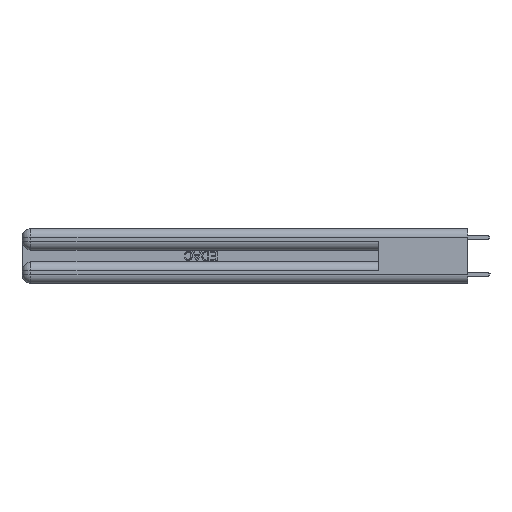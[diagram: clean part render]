
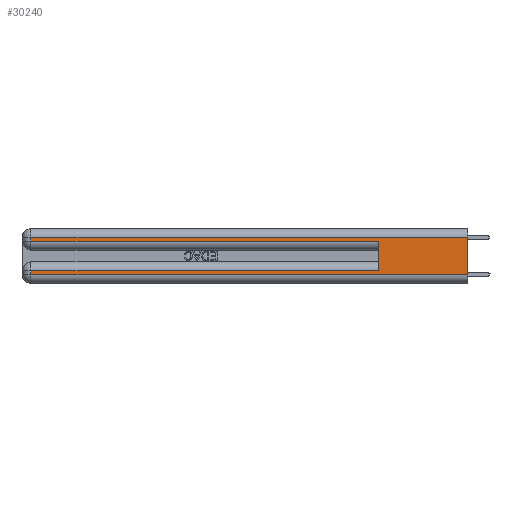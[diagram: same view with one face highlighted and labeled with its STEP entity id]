
A CAD part, left-side view. The second image highlights one B-rep face of the part: STEP entity #30240.
In plain terms, the highlighted planar face has unit normal (-1, 0, 0).
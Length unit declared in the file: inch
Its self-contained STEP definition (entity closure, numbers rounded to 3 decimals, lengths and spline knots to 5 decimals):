
#7 = CARTESIAN_POINT ( 'NONE',  ( 0., 2.94, 0.37 ) ) ;
#3219 = CARTESIAN_POINT ( 'NONE',  ( 0., 0., 0.085 ) ) ;
#3755 = EDGE_CURVE ( 'NONE', #18527, #27031, #7612, .T. ) ;
#4106 = AXIS2_PLACEMENT_3D ( 'NONE', #27947, #5730, #11053 ) ;
#4420 = CARTESIAN_POINT ( 'NONE',  ( 0., 2.94, 0.285 ) ) ;
#5433 = EDGE_CURVE ( 'NONE', #17912, #18527, #13097, .T. ) ;
#5436 = VECTOR ( 'NONE', #29998, 39.37008 ) ;
#5730 = DIRECTION ( 'NONE',  ( 1., 0., 0. ) ) ;
#5735 = CARTESIAN_POINT ( 'NONE',  ( 0., 2.94, 0.31 ) ) ;
#6537 = VECTOR ( 'NONE', #25739, 39.37008 ) ;
#6724 = DIRECTION ( 'NONE',  ( 0., -1., 0. ) ) ;
#6914 = EDGE_LOOP ( 'NONE', ( #13247, #14036, #29151, #11154, #9798, #8799, #14814, #30757 ) ) ;
#7612 = LINE ( 'NONE', #7, #22036 ) ;
#7779 = VECTOR ( 'NONE', #24035, 39.37008 ) ;
#7890 = VECTOR ( 'NONE', #28165, 39.37008 ) ;
#7951 = CARTESIAN_POINT ( 'NONE',  ( 0., 0., 0.31 ) ) ;
#8275 = LINE ( 'NONE', #7951, #5436 ) ;
#8799 = ORIENTED_EDGE ( 'NONE', *, *, #5433, .T. ) ;
#9798 = ORIENTED_EDGE ( 'NONE', *, *, #31322, .F. ) ;
#9923 = VERTEX_POINT ( 'NONE', #28962 ) ;
#10013 = CARTESIAN_POINT ( 'NONE',  ( 0., 2.94, 0.37 ) ) ;
#10562 = VERTEX_POINT ( 'NONE', #21533 ) ;
#11053 = DIRECTION ( 'NONE',  ( 0., 0., -1. ) ) ;
#11154 = ORIENTED_EDGE ( 'NONE', *, *, #29884, .T. ) ;
#12151 = EDGE_CURVE ( 'NONE', #27031, #10562, #17333, .T. ) ;
#12779 = DIRECTION ( 'NONE',  ( 0., 0., -1. ) ) ;
#13097 = LINE ( 'NONE', #3219, #6537 ) ;
#13236 = LINE ( 'NONE', #25394, #7890 ) ;
#13247 = ORIENTED_EDGE ( 'NONE', *, *, #23794, .F. ) ;
#13486 = FACE_OUTER_BOUND ( 'NONE', #6914, .T. ) ;
#13489 = VERTEX_POINT ( 'NONE', #31961 ) ;
#14008 = CARTESIAN_POINT ( 'NONE',  ( 0., 0., 0.285 ) ) ;
#14036 = ORIENTED_EDGE ( 'NONE', *, *, #27481, .T. ) ;
#14279 = CARTESIAN_POINT ( 'NONE',  ( 0., 0., 0.06 ) ) ;
#14561 = VERTEX_POINT ( 'NONE', #5735 ) ;
#14814 = ORIENTED_EDGE ( 'NONE', *, *, #3755, .T. ) ;
#15209 = EDGE_CURVE ( 'NONE', #14561, #22999, #19588, .T. ) ;
#16082 = CARTESIAN_POINT ( 'NONE',  ( 0., 2.94, 0.085 ) ) ;
#17333 = LINE ( 'NONE', #14279, #31464 ) ;
#17912 = VERTEX_POINT ( 'NONE', #22678 ) ;
#18527 = VERTEX_POINT ( 'NONE', #16082 ) ;
#19588 = LINE ( 'NONE', #10013, #20721 ) ;
#19607 = DIRECTION ( 'NONE',  ( 0., 0., -1. ) ) ;
#20479 = PLANE ( 'NONE',  #4106 ) ;
#20721 = VECTOR ( 'NONE', #12779, 39.37008 ) ;
#21533 = CARTESIAN_POINT ( 'NONE',  ( 0., 0., 0.06 ) ) ;
#22036 = VECTOR ( 'NONE', #19607, 39.37008 ) ;
#22073 = CARTESIAN_POINT ( 'NONE',  ( 0., 0.6, 0.145 ) ) ;
#22678 = CARTESIAN_POINT ( 'NONE',  ( 0., 0.6, 0.085 ) ) ;
#22899 = CARTESIAN_POINT ( 'NONE',  ( 0., 2.94, 0.06 ) ) ;
#22999 = VERTEX_POINT ( 'NONE', #4420 ) ;
#23243 = VECTOR ( 'NONE', #6724, 39.37008 ) ;
#23794 = EDGE_CURVE ( 'NONE', #13489, #10562, #13236, .T. ) ;
#24035 = DIRECTION ( 'NONE',  ( 0., 0., 1. ) ) ;
#24648 = DIRECTION ( 'NONE',  ( 0., -1., 0. ) ) ;
#25394 = CARTESIAN_POINT ( 'NONE',  ( 0., 0., 0.37 ) ) ;
#25739 = DIRECTION ( 'NONE',  ( 0., 1., 0. ) ) ;
#27031 = VERTEX_POINT ( 'NONE', #22899 ) ;
#27481 = EDGE_CURVE ( 'NONE', #13489, #14561, #8275, .T. ) ;
#27947 = CARTESIAN_POINT ( 'NONE',  ( 0., 0., 0.37 ) ) ;
#28165 = DIRECTION ( 'NONE',  ( 0., 0., -1. ) ) ;
#28962 = CARTESIAN_POINT ( 'NONE',  ( 0., 0.6, 0.285 ) ) ;
#29151 = ORIENTED_EDGE ( 'NONE', *, *, #15209, .T. ) ;
#29217 = LINE ( 'NONE', #22073, #7779 ) ;
#29884 = EDGE_CURVE ( 'NONE', #22999, #9923, #31376, .T. ) ;
#29998 = DIRECTION ( 'NONE',  ( 0., 1., 0. ) ) ;
#30240 = ADVANCED_FACE ( 'NONE', ( #13486 ), #20479, .F. ) ;
#30757 = ORIENTED_EDGE ( 'NONE', *, *, #12151, .T. ) ;
#31322 = EDGE_CURVE ( 'NONE', #17912, #9923, #29217, .T. ) ;
#31376 = LINE ( 'NONE', #14008, #23243 ) ;
#31464 = VECTOR ( 'NONE', #24648, 39.37008 ) ;
#31961 = CARTESIAN_POINT ( 'NONE',  ( 0., 0., 0.31 ) ) ;
